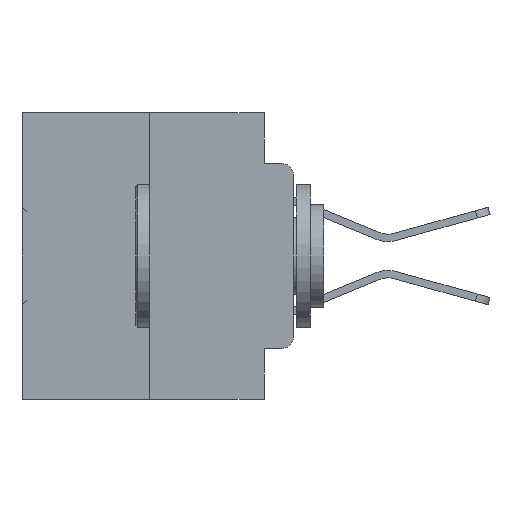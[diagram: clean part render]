
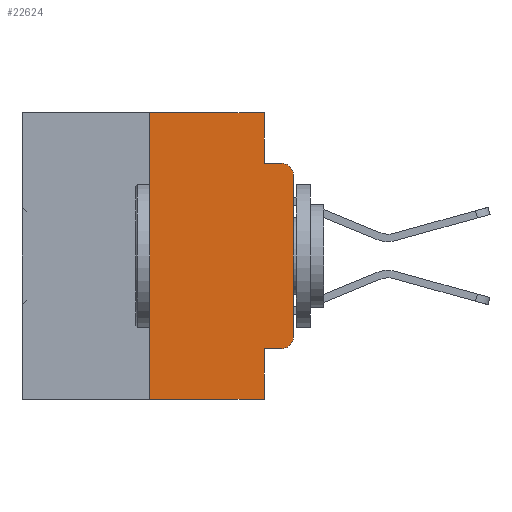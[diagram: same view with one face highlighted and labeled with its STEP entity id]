
A CAD part, left-side view. The second image highlights one B-rep face of the part: STEP entity #22624.
In plain terms, the highlighted planar face has unit normal (-1, 0, 0).
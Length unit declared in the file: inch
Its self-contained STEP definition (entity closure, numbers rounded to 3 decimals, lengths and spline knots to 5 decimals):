
#56 = VERTEX_POINT ( 'NONE', #4799 ) ;
#261 = CARTESIAN_POINT ( 'NONE',  ( 0., 0.02, -0.1085 ) ) ;
#357 = AXIS2_PLACEMENT_3D ( 'NONE', #19885, #23599, #22772 ) ;
#838 = VECTOR ( 'NONE', #1891, 39.37008 ) ;
#1298 = ORIENTED_EDGE ( 'NONE', *, *, #4211, .F. ) ;
#1401 = FACE_OUTER_BOUND ( 'NONE', #3600, .T. ) ;
#1691 = CARTESIAN_POINT ( 'NONE',  ( 0., 0., -0.3915 ) ) ;
#1891 = DIRECTION ( 'NONE',  ( 0., -1., 0. ) ) ;
#2151 = CARTESIAN_POINT ( 'NONE',  ( 0., 0.051, -0.5 ) ) ;
#2520 = LINE ( 'NONE', #15858, #20931 ) ;
#3025 = DIRECTION ( 'NONE',  ( 0., 0., 1. ) ) ;
#3067 = ORIENTED_EDGE ( 'NONE', *, *, #31264, .T. ) ;
#3600 = EDGE_LOOP ( 'NONE', ( #26451, #3067, #29552, #1298, #23438, #16158, #20294, #6163, #30501, #28782 ) ) ;
#3629 = EDGE_CURVE ( 'NONE', #9834, #21656, #16669, .T. ) ;
#4211 = EDGE_CURVE ( 'NONE', #56, #9834, #26454, .T. ) ;
#4741 = LINE ( 'NONE', #7630, #22956 ) ;
#4799 = CARTESIAN_POINT ( 'NONE',  ( 0., 0.051, 0. ) ) ;
#6163 = ORIENTED_EDGE ( 'NONE', *, *, #28778, .F. ) ;
#7078 = VERTEX_POINT ( 'NONE', #16680 ) ;
#7457 = DIRECTION ( 'NONE',  ( 0., -1., 0. ) ) ;
#7630 = CARTESIAN_POINT ( 'NONE',  ( 0., 0.051, -0.4115 ) ) ;
#7798 = CARTESIAN_POINT ( 'NONE',  ( 0., 0.473, 0. ) ) ;
#9469 = CARTESIAN_POINT ( 'NONE',  ( 0., 0.02, -0.0885 ) ) ;
#9834 = VERTEX_POINT ( 'NONE', #11075 ) ;
#10195 = EDGE_CURVE ( 'NONE', #20147, #25058, #4741, .T. ) ;
#10797 = CIRCLE ( 'NONE', #30889, 0.02 ) ;
#11075 = CARTESIAN_POINT ( 'NONE',  ( 0., 0.051, -0.0885 ) ) ;
#11685 = PLANE ( 'NONE',  #32186 ) ;
#12044 = CARTESIAN_POINT ( 'NONE',  ( 0., 0.473, 0. ) ) ;
#14309 = DIRECTION ( 'NONE',  ( -1., 0., 0. ) ) ;
#14528 = VERTEX_POINT ( 'NONE', #23933 ) ;
#14764 = LINE ( 'NONE', #23374, #21084 ) ;
#14796 = CARTESIAN_POINT ( 'NONE',  ( 0., 0.25, -0.5 ) ) ;
#15509 = CARTESIAN_POINT ( 'NONE',  ( 0., 0.051, 0. ) ) ;
#15858 = CARTESIAN_POINT ( 'NONE',  ( 0., 0.25, 0. ) ) ;
#16158 = ORIENTED_EDGE ( 'NONE', *, *, #25793, .F. ) ;
#16669 = LINE ( 'NONE', #24416, #20059 ) ;
#16680 = CARTESIAN_POINT ( 'NONE',  ( 0., 0.25, 0. ) ) ;
#18774 = DIRECTION ( 'NONE',  ( 0., -1., 0. ) ) ;
#19885 = CARTESIAN_POINT ( 'NONE',  ( 0., 0.02, -0.3915 ) ) ;
#20059 = VECTOR ( 'NONE', #27443, 39.37008 ) ;
#20147 = VERTEX_POINT ( 'NONE', #30366 ) ;
#20294 = ORIENTED_EDGE ( 'NONE', *, *, #24446, .T. ) ;
#20716 = DIRECTION ( 'NONE',  ( 0., 0., -1. ) ) ;
#20931 = VECTOR ( 'NONE', #26443, 39.37008 ) ;
#21084 = VECTOR ( 'NONE', #34300, 39.37008 ) ;
#21656 = VERTEX_POINT ( 'NONE', #9469 ) ;
#22624 = ADVANCED_FACE ( 'NONE', ( #1401 ), #11685, .F. ) ;
#22772 = DIRECTION ( 'NONE',  ( 0., 0., -1. ) ) ;
#22956 = VECTOR ( 'NONE', #7457, 39.37008 ) ;
#22997 = LINE ( 'NONE', #33928, #29950 ) ;
#23166 = DIRECTION ( 'NONE',  ( 1., 0., 0. ) ) ;
#23374 = CARTESIAN_POINT ( 'NONE',  ( 0., 0.051, 0. ) ) ;
#23438 = ORIENTED_EDGE ( 'NONE', *, *, #30282, .F. ) ;
#23599 = DIRECTION ( 'NONE',  ( -1., 0., 0. ) ) ;
#23933 = CARTESIAN_POINT ( 'NONE',  ( 0., 0., -0.1085 ) ) ;
#24416 = CARTESIAN_POINT ( 'NONE',  ( 0., 0.051, -0.0885 ) ) ;
#24446 = EDGE_CURVE ( 'NONE', #25646, #35176, #29225, .T. ) ;
#25058 = VERTEX_POINT ( 'NONE', #27713 ) ;
#25646 = VERTEX_POINT ( 'NONE', #14796 ) ;
#25758 = VECTOR ( 'NONE', #18774, 39.37008 ) ;
#25793 = EDGE_CURVE ( 'NONE', #25646, #7078, #2520, .T. ) ;
#26027 = DIRECTION ( 'NONE',  ( 0., 0., -1. ) ) ;
#26443 = DIRECTION ( 'NONE',  ( 0., 0., 1. ) ) ;
#26451 = ORIENTED_EDGE ( 'NONE', *, *, #35388, .T. ) ;
#26454 = LINE ( 'NONE', #15509, #27589 ) ;
#26697 = VERTEX_POINT ( 'NONE', #1691 ) ;
#27443 = DIRECTION ( 'NONE',  ( 0., -1., 0. ) ) ;
#27589 = VECTOR ( 'NONE', #20716, 39.37008 ) ;
#27713 = CARTESIAN_POINT ( 'NONE',  ( 0., 0.02, -0.4115 ) ) ;
#28366 = EDGE_CURVE ( 'NONE', #25058, #26697, #31372, .T. ) ;
#28778 = EDGE_CURVE ( 'NONE', #20147, #35176, #14764, .T. ) ;
#28782 = ORIENTED_EDGE ( 'NONE', *, *, #28366, .T. ) ;
#29225 = LINE ( 'NONE', #35120, #838 ) ;
#29552 = ORIENTED_EDGE ( 'NONE', *, *, #3629, .F. ) ;
#29950 = VECTOR ( 'NONE', #3025, 39.37008 ) ;
#30282 = EDGE_CURVE ( 'NONE', #7078, #56, #34729, .T. ) ;
#30366 = CARTESIAN_POINT ( 'NONE',  ( 0., 0.051, -0.4115 ) ) ;
#30501 = ORIENTED_EDGE ( 'NONE', *, *, #10195, .T. ) ;
#30889 = AXIS2_PLACEMENT_3D ( 'NONE', #261, #14309, #33151 ) ;
#31264 = EDGE_CURVE ( 'NONE', #14528, #21656, #10797, .T. ) ;
#31372 = CIRCLE ( 'NONE', #357, 0.02 ) ;
#32186 = AXIS2_PLACEMENT_3D ( 'NONE', #12044, #23166, #26027 ) ;
#33151 = DIRECTION ( 'NONE',  ( 0., 0., -1. ) ) ;
#33928 = CARTESIAN_POINT ( 'NONE',  ( 0., 0., 0. ) ) ;
#34300 = DIRECTION ( 'NONE',  ( 0., 0., -1. ) ) ;
#34729 = LINE ( 'NONE', #7798, #25758 ) ;
#35120 = CARTESIAN_POINT ( 'NONE',  ( 0., 0.473, -0.5 ) ) ;
#35176 = VERTEX_POINT ( 'NONE', #2151 ) ;
#35388 = EDGE_CURVE ( 'NONE', #26697, #14528, #22997, .T. ) ;
